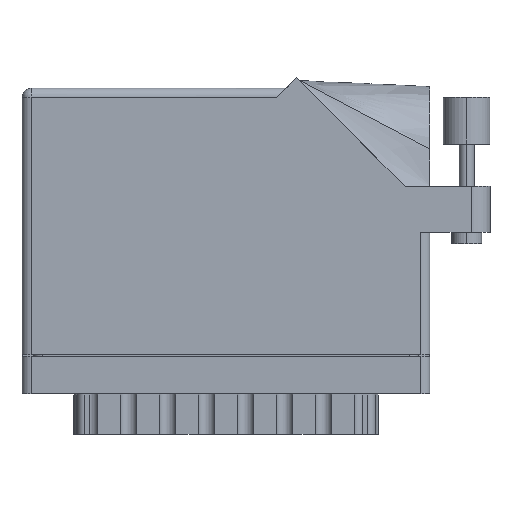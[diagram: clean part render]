
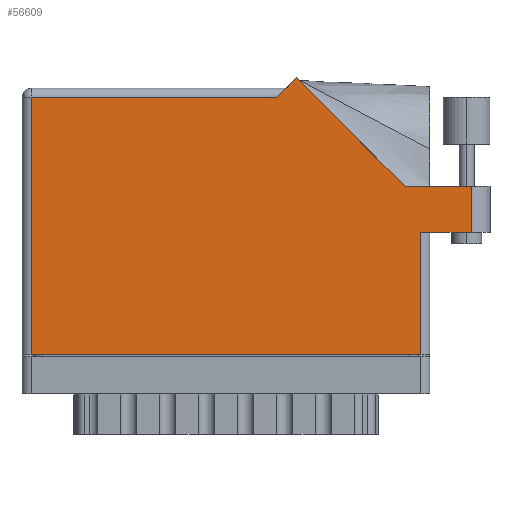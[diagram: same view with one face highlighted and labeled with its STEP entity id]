
A CAD part, front view. The second image highlights one B-rep face of the part: STEP entity #56609.
In plain terms, the highlighted face is planar.
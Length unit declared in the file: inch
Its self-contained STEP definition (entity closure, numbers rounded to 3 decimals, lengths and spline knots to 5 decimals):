
#713 = CARTESIAN_POINT ( 'NONE',  ( 2.993, 1.122, 0. ) ) ;
#1067 = LINE ( 'NONE', #38259, #8796 ) ;
#1293 = CARTESIAN_POINT ( 'NONE',  ( 1.82871, 1.84571, 0. ) ) ;
#2257 = ORIENTED_EDGE ( 'NONE', *, *, #17474, .T. ) ;
#2301 = AXIS2_PLACEMENT_3D ( 'NONE', #9261, #14771, #31984 ) ;
#2717 = DIRECTION ( 'NONE',  ( 0., -1., 0. ) ) ;
#3062 = ORIENTED_EDGE ( 'NONE', *, *, #48310, .T. ) ;
#4892 = PLANE ( 'NONE',  #2301 ) ;
#5141 = VECTOR ( 'NONE', #25780, 39.37008 ) ;
#5393 = DIRECTION ( 'NONE',  ( -1., 0., 0. ) ) ;
#6956 = EDGE_CURVE ( 'NONE', #8184, #45987, #52478, .T. ) ;
#8184 = VERTEX_POINT ( 'NONE', #11290 ) ;
#8703 = ORIENTED_EDGE ( 'NONE', *, *, #37196, .T. ) ;
#8796 = VECTOR ( 'NONE', #5393, 39.37008 ) ;
#9261 = CARTESIAN_POINT ( 'NONE',  ( 0., 1.775, 0. ) ) ;
#10657 = VECTOR ( 'NONE', #70764, 39.37008 ) ;
#10859 = VERTEX_POINT ( 'NONE', #22689 ) ;
#11290 = CARTESIAN_POINT ( 'NONE',  ( 2.656, 0.815, 0. ) ) ;
#12529 = DIRECTION ( 'NONE',  ( 1., 0., 0. ) ) ;
#12857 = EDGE_CURVE ( 'NONE', #34311, #33030, #1067, .T. ) ;
#13780 = CARTESIAN_POINT ( 'NONE',  ( 0.062, 0., 0. ) ) ;
#14771 = DIRECTION ( 'NONE',  ( 0., 0., -1. ) ) ;
#16201 = CARTESIAN_POINT ( 'NONE',  ( 2.656, 0., 0. ) ) ;
#17403 = ORIENTED_EDGE ( 'NONE', *, *, #12857, .T. ) ;
#17474 = EDGE_CURVE ( 'NONE', #10859, #56745, #21791, .T. ) ;
#20646 = EDGE_LOOP ( 'NONE', ( #42891, #8703, #3062, #67173, #21290, #17403, #62334, #2257, #35747 ) ) ;
#21290 = ORIENTED_EDGE ( 'NONE', *, *, #65223, .T. ) ;
#21791 = LINE ( 'NONE', #38067, #10657 ) ;
#22689 = CARTESIAN_POINT ( 'NONE',  ( 0.062, 0., 0. ) ) ;
#24146 = VECTOR ( 'NONE', #12529, 39.37008 ) ;
#24636 = LINE ( 'NONE', #713, #45178 ) ;
#25267 = CARTESIAN_POINT ( 'NONE',  ( 2.656, 0.815, 0. ) ) ;
#25780 = DIRECTION ( 'NONE',  ( -0.707, -0.707, 0. ) ) ;
#28505 = DIRECTION ( 'NONE',  ( -0.707, 0.707, 0. ) ) ;
#30541 = VECTOR ( 'NONE', #2717, 39.37008 ) ;
#31984 = DIRECTION ( 'NONE',  ( -1., 0., 0. ) ) ;
#32258 = CARTESIAN_POINT ( 'NONE',  ( 2.993, 1.122, 0. ) ) ;
#33030 = VERTEX_POINT ( 'NONE', #57106 ) ;
#34016 = LINE ( 'NONE', #13780, #30541 ) ;
#34311 = VERTEX_POINT ( 'NONE', #46846 ) ;
#35747 = ORIENTED_EDGE ( 'NONE', *, *, #68373, .T. ) ;
#36009 = EDGE_CURVE ( 'NONE', #61173, #69285, #52279, .T. ) ;
#37196 = EDGE_CURVE ( 'NONE', #45987, #52436, #24636, .T. ) ;
#38067 = CARTESIAN_POINT ( 'NONE',  ( 0., 0., 0. ) ) ;
#38259 = CARTESIAN_POINT ( 'NONE',  ( 0., 1.713, 0. ) ) ;
#39434 = VECTOR ( 'NONE', #28505, 39.37008 ) ;
#39855 = LINE ( 'NONE', #25267, #50985 ) ;
#41673 = DIRECTION ( 'NONE',  ( -1., 0., 0. ) ) ;
#42775 = CARTESIAN_POINT ( 'NONE',  ( 1.758, 1.775, 0. ) ) ;
#42891 = ORIENTED_EDGE ( 'NONE', *, *, #6956, .T. ) ;
#44699 = CARTESIAN_POINT ( 'NONE',  ( 2.993, 0.815, 0. ) ) ;
#45178 = VECTOR ( 'NONE', #55142, 39.37008 ) ;
#45987 = VERTEX_POINT ( 'NONE', #44699 ) ;
#46201 = EDGE_CURVE ( 'NONE', #33030, #10859, #34016, .T. ) ;
#46845 = FACE_OUTER_BOUND ( 'NONE', #20646, .T. ) ;
#46846 = CARTESIAN_POINT ( 'NONE',  ( 1.696, 1.713, 0. ) ) ;
#47404 = LINE ( 'NONE', #57278, #67078 ) ;
#48310 = EDGE_CURVE ( 'NONE', #52436, #61173, #47404, .T. ) ;
#48875 = LINE ( 'NONE', #42775, #5141 ) ;
#49198 = CARTESIAN_POINT ( 'NONE',  ( 2.718, 0.815, 0. ) ) ;
#50985 = VECTOR ( 'NONE', #61867, 39.37008 ) ;
#52279 = LINE ( 'NONE', #61317, #39434 ) ;
#52436 = VERTEX_POINT ( 'NONE', #32258 ) ;
#52478 = LINE ( 'NONE', #49198, #24146 ) ;
#55142 = DIRECTION ( 'NONE',  ( 0., 1., 0. ) ) ;
#56609 = ADVANCED_FACE ( 'NONE', ( #46845 ), #4892, .F. ) ;
#56745 = VERTEX_POINT ( 'NONE', #16201 ) ;
#57106 = CARTESIAN_POINT ( 'NONE',  ( 0.062, 1.713, 0. ) ) ;
#57278 = CARTESIAN_POINT ( 'NONE',  ( 3.118, 1.122, 0. ) ) ;
#57751 = CARTESIAN_POINT ( 'NONE',  ( 2.55242, 1.122, 0. ) ) ;
#61173 = VERTEX_POINT ( 'NONE', #57751 ) ;
#61317 = CARTESIAN_POINT ( 'NONE',  ( 2.55242, 1.122, 0. ) ) ;
#61867 = DIRECTION ( 'NONE',  ( 0., 1., 0. ) ) ;
#62334 = ORIENTED_EDGE ( 'NONE', *, *, #46201, .T. ) ;
#65223 = EDGE_CURVE ( 'NONE', #69285, #34311, #48875, .T. ) ;
#67078 = VECTOR ( 'NONE', #41673, 39.37008 ) ;
#67173 = ORIENTED_EDGE ( 'NONE', *, *, #36009, .T. ) ;
#68373 = EDGE_CURVE ( 'NONE', #56745, #8184, #39855, .T. ) ;
#69285 = VERTEX_POINT ( 'NONE', #1293 ) ;
#70764 = DIRECTION ( 'NONE',  ( 1., 0., 0. ) ) ;
